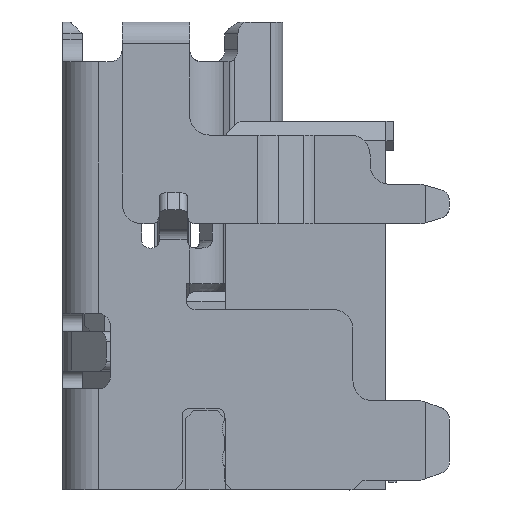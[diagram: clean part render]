
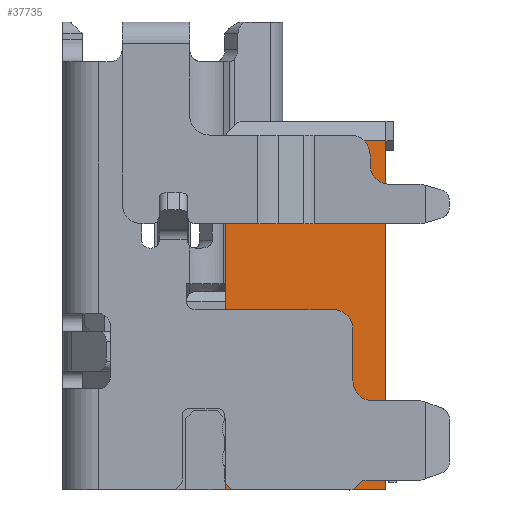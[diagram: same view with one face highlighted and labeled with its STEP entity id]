
A CAD part, left-side view. The second image highlights one B-rep face of the part: STEP entity #37735.
In plain terms, the highlighted planar face has unit normal (-1, 0, 0).
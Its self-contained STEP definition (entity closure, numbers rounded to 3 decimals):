
#1549 = EDGE_CURVE ( 'NONE', #55325, #15473, #74545, .T. ) ;
#2258 = ORIENTED_EDGE ( 'NONE', *, *, #98622, .F. ) ;
#5984 = VECTOR ( 'NONE', #102664, 1000. ) ;
#9106 = CARTESIAN_POINT ( 'NONE',  ( -6.95, -7.625, -0.5 ) ) ;
#12800 = DIRECTION ( 'NONE',  ( 0., 0., -1. ) ) ;
#15473 = VERTEX_POINT ( 'NONE', #39342 ) ;
#16423 = CARTESIAN_POINT ( 'NONE',  ( -6.95, -3.575, -6.9 ) ) ;
#18683 = VERTEX_POINT ( 'NONE', #92944 ) ;
#20322 = EDGE_CURVE ( 'NONE', #18683, #51009, #86404, .T. ) ;
#23324 = LINE ( 'NONE', #67897, #98382 ) ;
#25087 = LINE ( 'NONE', #16423, #99542 ) ;
#27672 = CARTESIAN_POINT ( 'NONE',  ( -6.95, -5.6, -0.5 ) ) ;
#29377 = EDGE_LOOP ( 'NONE', ( #106466, #2258, #67492, #111448, #88797 ) ) ;
#30938 = LINE ( 'NONE', #27672, #104659 ) ;
#31303 = FACE_OUTER_BOUND ( 'NONE', #29377, .T. ) ;
#37735 = ADVANCED_FACE ( 'NONE', ( #31303 ), #101920, .F. ) ;
#39342 = CARTESIAN_POINT ( 'NONE',  ( -6.95, -7.625, -9.3 ) ) ;
#40927 = CARTESIAN_POINT ( 'NONE',  ( -6.95, -7.625, -4.9 ) ) ;
#41489 = DIRECTION ( 'NONE',  ( 0., 0., -1. ) ) ;
#46516 = VECTOR ( 'NONE', #41489, 1000. ) ;
#51009 = VERTEX_POINT ( 'NONE', #64390 ) ;
#51081 = CARTESIAN_POINT ( 'NONE',  ( -6.95, -3.575, -4.9 ) ) ;
#55325 = VERTEX_POINT ( 'NONE', #9106 ) ;
#58634 = DIRECTION ( 'NONE',  ( 0., 1., 0. ) ) ;
#61325 = VERTEX_POINT ( 'NONE', #92740 ) ;
#64390 = CARTESIAN_POINT ( 'NONE',  ( -6.95, -3.575, -0.5 ) ) ;
#66790 = EDGE_CURVE ( 'NONE', #51009, #55325, #30938, .T. ) ;
#67492 = ORIENTED_EDGE ( 'NONE', *, *, #1549, .F. ) ;
#67897 = CARTESIAN_POINT ( 'NONE',  ( -6.95, -5.6, -9.3 ) ) ;
#74545 = LINE ( 'NONE', #40927, #46516 ) ;
#83599 = DIRECTION ( 'NONE',  ( 0., -1., 0. ) ) ;
#86404 = LINE ( 'NONE', #51081, #5984 ) ;
#88797 = ORIENTED_EDGE ( 'NONE', *, *, #20322, .F. ) ;
#92740 = CARTESIAN_POINT ( 'NONE',  ( -6.95, -3.575, -9.3 ) ) ;
#92944 = CARTESIAN_POINT ( 'NONE',  ( -6.95, -3.575, -4.5 ) ) ;
#94498 = EDGE_CURVE ( 'NONE', #18683, #61325, #25087, .T. ) ;
#95130 = DIRECTION ( 'NONE',  ( 0., 0., -1. ) ) ;
#98264 = AXIS2_PLACEMENT_3D ( 'NONE', #110608, #112300, #12800 ) ;
#98382 = VECTOR ( 'NONE', #58634, 1000. ) ;
#98622 = EDGE_CURVE ( 'NONE', #15473, #61325, #23324, .T. ) ;
#99542 = VECTOR ( 'NONE', #95130, 1000. ) ;
#101920 = PLANE ( 'NONE',  #98264 ) ;
#102664 = DIRECTION ( 'NONE',  ( 0., 0., 1. ) ) ;
#104659 = VECTOR ( 'NONE', #83599, 1000. ) ;
#106466 = ORIENTED_EDGE ( 'NONE', *, *, #94498, .T. ) ;
#110608 = CARTESIAN_POINT ( 'NONE',  ( -6.95, -5.6, -4.9 ) ) ;
#111448 = ORIENTED_EDGE ( 'NONE', *, *, #66790, .F. ) ;
#112300 = DIRECTION ( 'NONE',  ( 1., 0., 0. ) ) ;
